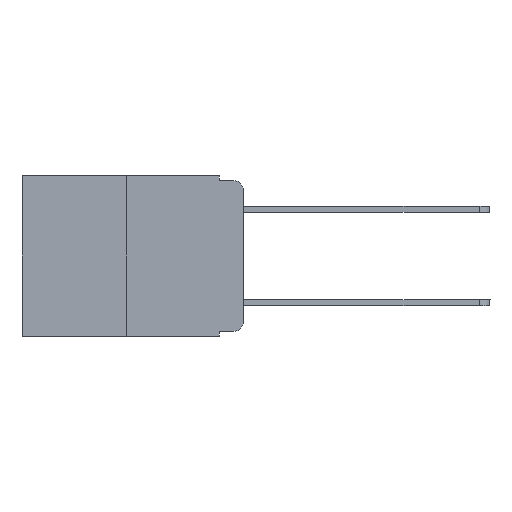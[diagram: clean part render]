
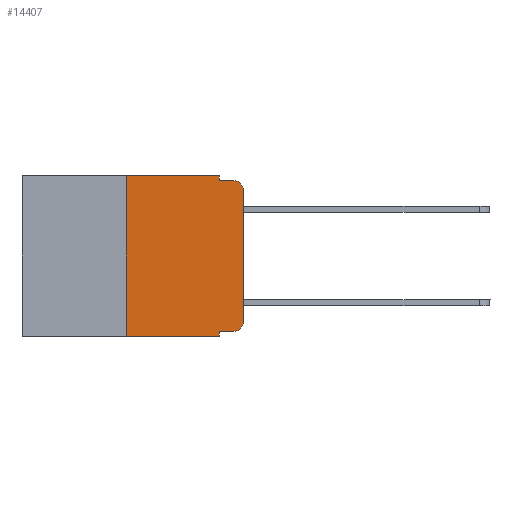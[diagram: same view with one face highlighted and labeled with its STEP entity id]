
A CAD part, left-side view. The second image highlights one B-rep face of the part: STEP entity #14407.
In plain terms, the highlighted planar face has unit normal (-1, 0, 0).
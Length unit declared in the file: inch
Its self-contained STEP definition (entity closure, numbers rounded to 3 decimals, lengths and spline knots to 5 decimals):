
#526 = ORIENTED_EDGE ( 'NONE', *, *, #1452, .F. ) ;
#1452 = EDGE_CURVE ( 'NONE', #8261, #2458, #6312, .T. ) ;
#1565 = CARTESIAN_POINT ( 'NONE',  ( 0., 0.02, -0.333 ) ) ;
#1615 = CARTESIAN_POINT ( 'NONE',  ( 0., 0.051, -0.333 ) ) ;
#1652 = DIRECTION ( 'NONE',  ( 0., 0., -1. ) ) ;
#1835 = CARTESIAN_POINT ( 'NONE',  ( 0., 0.02, -0.313 ) ) ;
#1869 = ORIENTED_EDGE ( 'NONE', *, *, #3082, .F. ) ;
#1874 = CARTESIAN_POINT ( 'NONE',  ( 0., 0.473, 0. ) ) ;
#2013 = CARTESIAN_POINT ( 'NONE',  ( 0., 0.051, -0.343 ) ) ;
#2294 = ORIENTED_EDGE ( 'NONE', *, *, #8334, .T. ) ;
#2314 = EDGE_CURVE ( 'NONE', #11935, #2488, #6474, .T. ) ;
#2365 = VERTEX_POINT ( 'NONE', #12680 ) ;
#2458 = VERTEX_POINT ( 'NONE', #2013 ) ;
#2488 = VERTEX_POINT ( 'NONE', #9417 ) ;
#2667 = DIRECTION ( 'NONE',  ( 0., 0., 1. ) ) ;
#2795 = CIRCLE ( 'NONE', #11185, 0.02 ) ;
#2968 = VERTEX_POINT ( 'NONE', #12980 ) ;
#2985 = CARTESIAN_POINT ( 'NONE',  ( 0., 0.051, -0.333 ) ) ;
#2991 = PLANE ( 'NONE',  #10514 ) ;
#3064 = DIRECTION ( 'NONE',  ( -1., 0., 0. ) ) ;
#3082 = EDGE_CURVE ( 'NONE', #2488, #2365, #13355, .T. ) ;
#3547 = FACE_OUTER_BOUND ( 'NONE', #8476, .T. ) ;
#3917 = CARTESIAN_POINT ( 'NONE',  ( 0., 0., 0. ) ) ;
#4102 = DIRECTION ( 'NONE',  ( 0., 0., -1. ) ) ;
#4418 = VECTOR ( 'NONE', #2667, 39.37008 ) ;
#4725 = CARTESIAN_POINT ( 'NONE',  ( 0., 0.051, -0.01 ) ) ;
#4998 = CARTESIAN_POINT ( 'NONE',  ( 0., 0.473, 0. ) ) ;
#5079 = EDGE_CURVE ( 'NONE', #9464, #2968, #10133, .T. ) ;
#5098 = ORIENTED_EDGE ( 'NONE', *, *, #13923, .T. ) ;
#5581 = ORIENTED_EDGE ( 'NONE', *, *, #11830, .T. ) ;
#5743 = VECTOR ( 'NONE', #5957, 39.37008 ) ;
#5845 = CARTESIAN_POINT ( 'NONE',  ( 0., 0.473, -0.343 ) ) ;
#5957 = DIRECTION ( 'NONE',  ( 0., -1., 0. ) ) ;
#6016 = VECTOR ( 'NONE', #15550, 39.37008 ) ;
#6084 = VECTOR ( 'NONE', #7644, 39.37008 ) ;
#6293 = VECTOR ( 'NONE', #4102, 39.37008 ) ;
#6312 = LINE ( 'NONE', #9147, #15700 ) ;
#6474 = LINE ( 'NONE', #11494, #10099 ) ;
#7300 = CARTESIAN_POINT ( 'NONE',  ( 0., 0.25, -0.343 ) ) ;
#7362 = CIRCLE ( 'NONE', #9189, 0.02 ) ;
#7569 = ORIENTED_EDGE ( 'NONE', *, *, #5079, .F. ) ;
#7644 = DIRECTION ( 'NONE',  ( 0., -1., 0. ) ) ;
#7823 = DIRECTION ( 'NONE',  ( 0., 0., -1. ) ) ;
#7966 = ORIENTED_EDGE ( 'NONE', *, *, #8074, .T. ) ;
#8029 = DIRECTION ( 'NONE',  ( 0., 0., -1. ) ) ;
#8074 = EDGE_CURVE ( 'NONE', #8261, #10973, #13859, .T. ) ;
#8261 = VERTEX_POINT ( 'NONE', #1615 ) ;
#8334 = EDGE_CURVE ( 'NONE', #10973, #11814, #7362, .T. ) ;
#8476 = EDGE_LOOP ( 'NONE', ( #15778, #5098, #7569, #13122, #1869, #10787, #5581, #526, #7966, #2294 ) ) ;
#8580 = CARTESIAN_POINT ( 'NONE',  ( 0., 0., -0.03 ) ) ;
#8727 = CARTESIAN_POINT ( 'NONE',  ( 0., 0.02, -0.03 ) ) ;
#9147 = CARTESIAN_POINT ( 'NONE',  ( 0., 0.051, 0. ) ) ;
#9189 = AXIS2_PLACEMENT_3D ( 'NONE', #1835, #3064, #7823 ) ;
#9417 = CARTESIAN_POINT ( 'NONE',  ( 0., 0.25, 0. ) ) ;
#9464 = VERTEX_POINT ( 'NONE', #4725 ) ;
#9764 = CARTESIAN_POINT ( 'NONE',  ( 0., 0.051, -0.01 ) ) ;
#9932 = EDGE_CURVE ( 'NONE', #11814, #11220, #15554, .T. ) ;
#10099 = VECTOR ( 'NONE', #15629, 39.37008 ) ;
#10133 = LINE ( 'NONE', #9764, #13193 ) ;
#10514 = AXIS2_PLACEMENT_3D ( 'NONE', #1874, #15138, #1652 ) ;
#10787 = ORIENTED_EDGE ( 'NONE', *, *, #2314, .F. ) ;
#10973 = VERTEX_POINT ( 'NONE', #1565 ) ;
#11185 = AXIS2_PLACEMENT_3D ( 'NONE', #8727, #14950, #13592 ) ;
#11220 = VERTEX_POINT ( 'NONE', #8580 ) ;
#11456 = CARTESIAN_POINT ( 'NONE',  ( 0., 0.051, 0. ) ) ;
#11494 = CARTESIAN_POINT ( 'NONE',  ( 0., 0.25, 0. ) ) ;
#11814 = VERTEX_POINT ( 'NONE', #15642 ) ;
#11830 = EDGE_CURVE ( 'NONE', #11935, #2458, #14951, .T. ) ;
#11935 = VERTEX_POINT ( 'NONE', #7300 ) ;
#12680 = CARTESIAN_POINT ( 'NONE',  ( 0., 0.051, 0. ) ) ;
#12980 = CARTESIAN_POINT ( 'NONE',  ( 0., 0.02, -0.01 ) ) ;
#13005 = LINE ( 'NONE', #11456, #6293 ) ;
#13122 = ORIENTED_EDGE ( 'NONE', *, *, #13400, .F. ) ;
#13193 = VECTOR ( 'NONE', #14650, 39.37008 ) ;
#13355 = LINE ( 'NONE', #4998, #6084 ) ;
#13400 = EDGE_CURVE ( 'NONE', #2365, #9464, #13005, .T. ) ;
#13592 = DIRECTION ( 'NONE',  ( 0., 0., -1. ) ) ;
#13859 = LINE ( 'NONE', #2985, #6016 ) ;
#13923 = EDGE_CURVE ( 'NONE', #11220, #2968, #2795, .T. ) ;
#14407 = ADVANCED_FACE ( 'NONE', ( #3547 ), #2991, .F. ) ;
#14650 = DIRECTION ( 'NONE',  ( 0., -1., 0. ) ) ;
#14950 = DIRECTION ( 'NONE',  ( -1., 0., 0. ) ) ;
#14951 = LINE ( 'NONE', #5845, #5743 ) ;
#15138 = DIRECTION ( 'NONE',  ( 1., 0., 0. ) ) ;
#15550 = DIRECTION ( 'NONE',  ( 0., -1., 0. ) ) ;
#15554 = LINE ( 'NONE', #3917, #4418 ) ;
#15629 = DIRECTION ( 'NONE',  ( 0., 0., 1. ) ) ;
#15642 = CARTESIAN_POINT ( 'NONE',  ( 0., 0., -0.313 ) ) ;
#15700 = VECTOR ( 'NONE', #8029, 39.37008 ) ;
#15778 = ORIENTED_EDGE ( 'NONE', *, *, #9932, .T. ) ;
